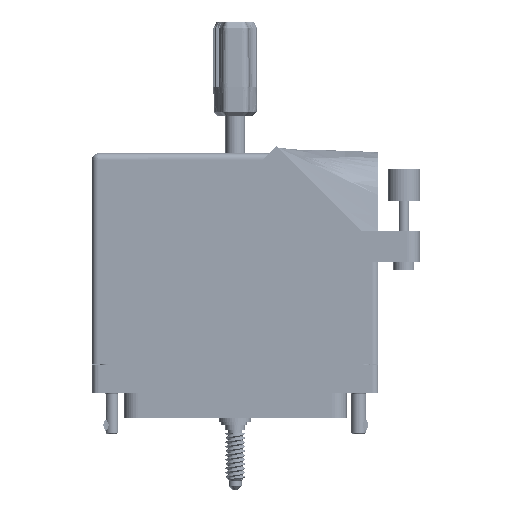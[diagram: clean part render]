
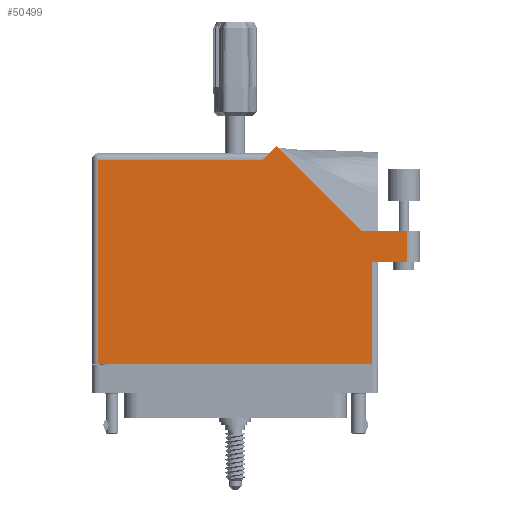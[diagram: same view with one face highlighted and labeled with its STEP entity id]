
A CAD part, front view. The second image highlights one B-rep face of the part: STEP entity #50499.
In plain terms, the highlighted face is planar.
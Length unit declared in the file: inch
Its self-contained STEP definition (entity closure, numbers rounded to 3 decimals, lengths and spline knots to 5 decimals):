
#431 = DIRECTION ( 'NONE',  ( 0., 1., 0. ) ) ;
#576 = ORIENTED_EDGE ( 'NONE', *, *, #37563, .T. ) ;
#5305 = LINE ( 'NONE', #62712, #83574 ) ;
#5672 = CARTESIAN_POINT ( 'NONE',  ( 1.3155, 0.88, 0.765 ) ) ;
#5900 = CARTESIAN_POINT ( 'NONE',  ( 0.39821, 2.00071, 0.765 ) ) ;
#7739 = VERTEX_POINT ( 'NONE', #112591 ) ;
#8901 = EDGE_CURVE ( 'NONE', #52455, #44555, #62096, .T. ) ;
#8916 = EDGE_CURVE ( 'NONE', #37133, #20860, #112383, .T. ) ;
#9471 = LINE ( 'NONE', #63406, #26328 ) ;
#13112 = VECTOR ( 'NONE', #28160, 39.37008 ) ;
#13562 = CARTESIAN_POINT ( 'NONE',  ( 1.3155, 0.88, 0.765 ) ) ;
#14371 = ORIENTED_EDGE ( 'NONE', *, *, #26741, .T. ) ;
#15397 = EDGE_CURVE ( 'NONE', #51884, #7739, #49768, .T. ) ;
#16767 = DIRECTION ( 'NONE',  ( 1., 0., 0. ) ) ;
#17500 = CARTESIAN_POINT ( 'NONE',  ( 1.6525, 0.88, 0.765 ) ) ;
#17756 = EDGE_LOOP ( 'NONE', ( #42589, #14371, #110742, #85758, #82184, #46273, #39748, #72631, #576 ) ) ;
#19548 = DIRECTION ( 'NONE',  ( 0., -1., 0. ) ) ;
#20860 = VERTEX_POINT ( 'NONE', #96066 ) ;
#26328 = VECTOR ( 'NONE', #71536, 39.37008 ) ;
#26511 = CARTESIAN_POINT ( 'NONE',  ( 1.6525, 1.187, 0.765 ) ) ;
#26741 = EDGE_CURVE ( 'NONE', #85870, #52455, #5305, .T. ) ;
#28160 = DIRECTION ( 'NONE',  ( -0.707, -0.707, 0. ) ) ;
#30419 = EDGE_CURVE ( 'NONE', #86688, #51884, #36938, .T. ) ;
#33526 = VECTOR ( 'NONE', #94769, 39.37008 ) ;
#36938 = LINE ( 'NONE', #109417, #13112 ) ;
#37133 = VERTEX_POINT ( 'NONE', #105860 ) ;
#37563 = EDGE_CURVE ( 'NONE', #20860, #38796, #83818, .T. ) ;
#38796 = VERTEX_POINT ( 'NONE', #13562 ) ;
#39748 = ORIENTED_EDGE ( 'NONE', *, *, #91761, .T. ) ;
#42589 = ORIENTED_EDGE ( 'NONE', *, *, #74703, .T. ) ;
#43680 = AXIS2_PLACEMENT_3D ( 'NONE', #50677, #86135, #58518 ) ;
#44555 = VERTEX_POINT ( 'NONE', #79450 ) ;
#46273 = ORIENTED_EDGE ( 'NONE', *, *, #15397, .T. ) ;
#49768 = LINE ( 'NONE', #79904, #94436 ) ;
#50499 = ADVANCED_FACE ( 'NONE', ( #86213 ), #86503, .F. ) ;
#50677 = CARTESIAN_POINT ( 'NONE',  ( -1.3775, 1.93, 0.765 ) ) ;
#51884 = VERTEX_POINT ( 'NONE', #72346 ) ;
#52095 = LINE ( 'NONE', #98067, #112158 ) ;
#52385 = CARTESIAN_POINT ( 'NONE',  ( 1.7775, 1.187, 0.765 ) ) ;
#52455 = VERTEX_POINT ( 'NONE', #26511 ) ;
#57927 = VECTOR ( 'NONE', #107004, 39.37008 ) ;
#58518 = DIRECTION ( 'NONE',  ( -1., 0., 0. ) ) ;
#62096 = LINE ( 'NONE', #52385, #57927 ) ;
#62712 = CARTESIAN_POINT ( 'NONE',  ( 1.6525, 1.187, 0.765 ) ) ;
#63406 = CARTESIAN_POINT ( 'NONE',  ( 1.21192, 1.187, 0.765 ) ) ;
#70195 = DIRECTION ( 'NONE',  ( -1., 0., 0. ) ) ;
#71445 = CARTESIAN_POINT ( 'NONE',  ( -1.3775, -0.1, 0.765 ) ) ;
#71536 = DIRECTION ( 'NONE',  ( -0.707, 0.707, 0. ) ) ;
#72346 = CARTESIAN_POINT ( 'NONE',  ( 0.2655, 1.868, 0.765 ) ) ;
#72631 = ORIENTED_EDGE ( 'NONE', *, *, #8916, .T. ) ;
#74703 = EDGE_CURVE ( 'NONE', #38796, #85870, #110108, .T. ) ;
#79450 = CARTESIAN_POINT ( 'NONE',  ( 1.21192, 1.187, 0.765 ) ) ;
#79904 = CARTESIAN_POINT ( 'NONE',  ( -1.3775, 1.868, 0.765 ) ) ;
#81979 = EDGE_CURVE ( 'NONE', #44555, #86688, #9471, .T. ) ;
#82184 = ORIENTED_EDGE ( 'NONE', *, *, #30419, .T. ) ;
#83574 = VECTOR ( 'NONE', #431, 39.37008 ) ;
#83818 = LINE ( 'NONE', #5672, #33526 ) ;
#85738 = VECTOR ( 'NONE', #16767, 39.37008 ) ;
#85758 = ORIENTED_EDGE ( 'NONE', *, *, #81979, .T. ) ;
#85870 = VERTEX_POINT ( 'NONE', #17500 ) ;
#86135 = DIRECTION ( 'NONE',  ( 0., 0., -1. ) ) ;
#86213 = FACE_OUTER_BOUND ( 'NONE', #17756, .T. ) ;
#86503 = PLANE ( 'NONE',  #43680 ) ;
#86688 = VERTEX_POINT ( 'NONE', #5900 ) ;
#91761 = EDGE_CURVE ( 'NONE', #7739, #37133, #52095, .T. ) ;
#94436 = VECTOR ( 'NONE', #70195, 39.37008 ) ;
#94769 = DIRECTION ( 'NONE',  ( 0., 1., 0. ) ) ;
#96066 = CARTESIAN_POINT ( 'NONE',  ( 1.3155, -0.1, 0.765 ) ) ;
#96167 = DIRECTION ( 'NONE',  ( 1., 0., 0. ) ) ;
#98067 = CARTESIAN_POINT ( 'NONE',  ( -1.3155, -0.1, 0.765 ) ) ;
#105860 = CARTESIAN_POINT ( 'NONE',  ( -1.3155, -0.1, 0.765 ) ) ;
#107004 = DIRECTION ( 'NONE',  ( -1., 0., 0. ) ) ;
#109417 = CARTESIAN_POINT ( 'NONE',  ( 0.3275, 1.93, 0.765 ) ) ;
#110108 = LINE ( 'NONE', #114919, #114368 ) ;
#110742 = ORIENTED_EDGE ( 'NONE', *, *, #8901, .T. ) ;
#112158 = VECTOR ( 'NONE', #19548, 39.37008 ) ;
#112383 = LINE ( 'NONE', #71445, #85738 ) ;
#112591 = CARTESIAN_POINT ( 'NONE',  ( -1.3155, 1.868, 0.765 ) ) ;
#114368 = VECTOR ( 'NONE', #96167, 39.37008 ) ;
#114919 = CARTESIAN_POINT ( 'NONE',  ( 1.3775, 0.88, 0.765 ) ) ;
